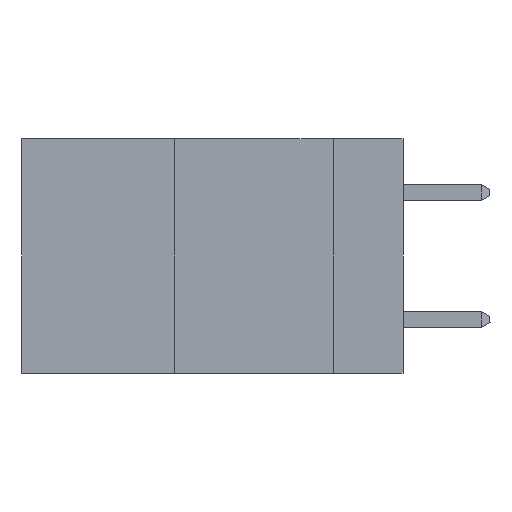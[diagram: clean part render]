
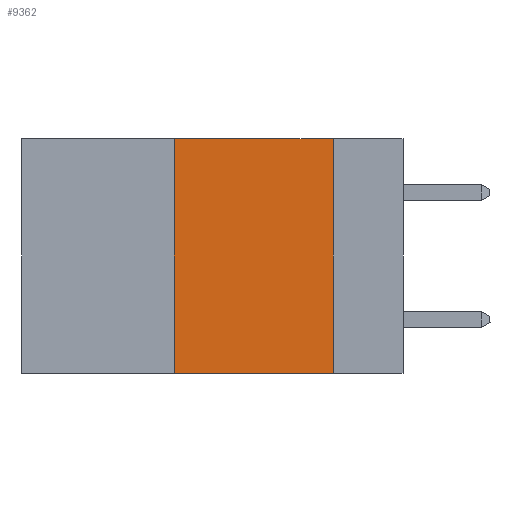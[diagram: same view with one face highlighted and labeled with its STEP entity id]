
A CAD part, left-side view. The second image highlights one B-rep face of the part: STEP entity #9362.
In plain terms, the highlighted planar face has unit normal (-1, 0, 0).
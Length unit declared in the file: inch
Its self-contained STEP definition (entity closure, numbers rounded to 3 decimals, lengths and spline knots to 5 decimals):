
#542 = CARTESIAN_POINT ( 'NONE',  ( 0., 0.11, 0. ) ) ;
#634 = DIRECTION ( 'NONE',  ( 0., 0., -1. ) ) ;
#720 = EDGE_LOOP ( 'NONE', ( #10398, #23685, #16524, #3718 ) ) ;
#1004 = CARTESIAN_POINT ( 'NONE',  ( 0., 0.36, 0. ) ) ;
#1368 = VERTEX_POINT ( 'NONE', #1004 ) ;
#1741 = VERTEX_POINT ( 'NONE', #10594 ) ;
#3718 = ORIENTED_EDGE ( 'NONE', *, *, #18257, .T. ) ;
#3764 = LINE ( 'NONE', #6020, #14065 ) ;
#4184 = VERTEX_POINT ( 'NONE', #6214 ) ;
#4349 = LINE ( 'NONE', #25846, #14344 ) ;
#4600 = PLANE ( 'NONE',  #22254 ) ;
#5389 = EDGE_CURVE ( 'NONE', #4184, #1368, #3764, .T. ) ;
#6020 = CARTESIAN_POINT ( 'NONE',  ( 0., 0.36, 0. ) ) ;
#6214 = CARTESIAN_POINT ( 'NONE',  ( 0., 0.36, -0.37 ) ) ;
#8008 = DIRECTION ( 'NONE',  ( 0., 0., 1. ) ) ;
#9362 = ADVANCED_FACE ( 'NONE', ( #22682 ), #4600, .F. ) ;
#10195 = LINE ( 'NONE', #17424, #14299 ) ;
#10398 = ORIENTED_EDGE ( 'NONE', *, *, #20401, .F. ) ;
#10520 = LINE ( 'NONE', #542, #25947 ) ;
#10594 = CARTESIAN_POINT ( 'NONE',  ( 0., 0.11, 0. ) ) ;
#11264 = CARTESIAN_POINT ( 'NONE',  ( 0., 0.11, -0.37 ) ) ;
#11744 = DIRECTION ( 'NONE',  ( 0., -1., 0. ) ) ;
#12523 = CARTESIAN_POINT ( 'NONE',  ( 0., 0.6, 0. ) ) ;
#12914 = EDGE_CURVE ( 'NONE', #1368, #1741, #10195, .T. ) ;
#14065 = VECTOR ( 'NONE', #8008, 39.37008 ) ;
#14299 = VECTOR ( 'NONE', #17259, 39.37008 ) ;
#14344 = VECTOR ( 'NONE', #11744, 39.37008 ) ;
#16524 = ORIENTED_EDGE ( 'NONE', *, *, #5389, .F. ) ;
#17259 = DIRECTION ( 'NONE',  ( 0., -1., 0. ) ) ;
#17424 = CARTESIAN_POINT ( 'NONE',  ( 0., 0.6, 0. ) ) ;
#18257 = EDGE_CURVE ( 'NONE', #4184, #25159, #4349, .T. ) ;
#18555 = DIRECTION ( 'NONE',  ( 1., 0., 0. ) ) ;
#20401 = EDGE_CURVE ( 'NONE', #1741, #25159, #10520, .T. ) ;
#20732 = DIRECTION ( 'NONE',  ( 0., 0., -1. ) ) ;
#22254 = AXIS2_PLACEMENT_3D ( 'NONE', #12523, #18555, #20732 ) ;
#22682 = FACE_OUTER_BOUND ( 'NONE', #720, .T. ) ;
#23685 = ORIENTED_EDGE ( 'NONE', *, *, #12914, .F. ) ;
#25159 = VERTEX_POINT ( 'NONE', #11264 ) ;
#25846 = CARTESIAN_POINT ( 'NONE',  ( 0., 0.6, -0.37 ) ) ;
#25947 = VECTOR ( 'NONE', #634, 39.37008 ) ;
